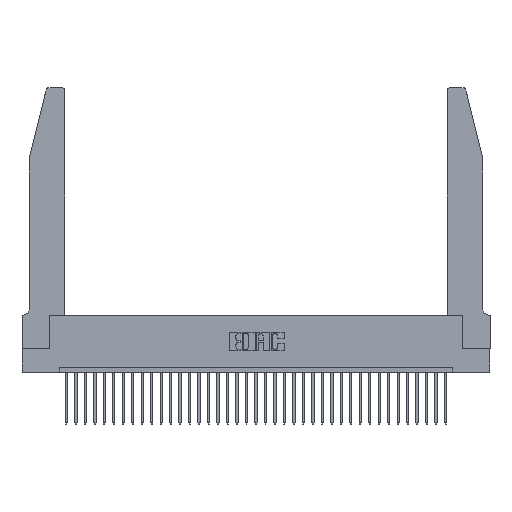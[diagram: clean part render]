
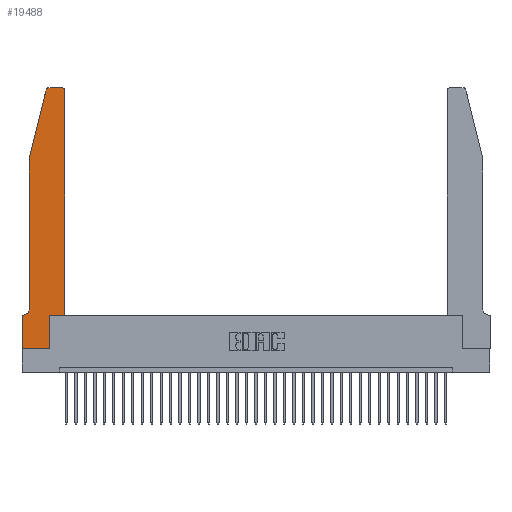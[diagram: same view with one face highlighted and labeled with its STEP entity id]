
A CAD part, top view. The second image highlights one B-rep face of the part: STEP entity #19488.
In plain terms, the highlighted planar face has unit normal (0, 0, 1).
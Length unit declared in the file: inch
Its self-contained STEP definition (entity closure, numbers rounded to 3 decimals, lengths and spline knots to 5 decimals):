
#226 = ORIENTED_EDGE ( 'NONE', *, *, #31575, .T. ) ;
#304 = LINE ( 'NONE', #4262, #28851 ) ;
#483 = LINE ( 'NONE', #24571, #19931 ) ;
#789 = DIRECTION ( 'NONE',  ( -1., 0., 0. ) ) ;
#846 = DIRECTION ( 'NONE',  ( -0.239, -0.971, 0. ) ) ;
#2002 = ORIENTED_EDGE ( 'NONE', *, *, #4133, .T. ) ;
#2169 = LINE ( 'NONE', #10040, #11622 ) ;
#2598 = ORIENTED_EDGE ( 'NONE', *, *, #31284, .T. ) ;
#2631 = CARTESIAN_POINT ( 'NONE',  ( 0., 0., 0.37 ) ) ;
#3411 = VECTOR ( 'NONE', #789, 39.37008 ) ;
#3444 = EDGE_CURVE ( 'NONE', #24111, #4495, #8761, .T. ) ;
#4103 = CARTESIAN_POINT ( 'NONE',  ( 0.2865, 0.35, 0.37 ) ) ;
#4133 = EDGE_CURVE ( 'NONE', #21514, #27555, #483, .T. ) ;
#4262 = CARTESIAN_POINT ( 'NONE',  ( 0.4505, 0.35, 0.37 ) ) ;
#4495 = VERTEX_POINT ( 'NONE', #30017 ) ;
#4595 = CARTESIAN_POINT ( 'NONE',  ( 0., 0., 0.37 ) ) ;
#5075 = VERTEX_POINT ( 'NONE', #26132 ) ;
#5099 = LINE ( 'NONE', #9094, #8101 ) ;
#6666 = DIRECTION ( 'NONE',  ( 0., 0., 1. ) ) ;
#6818 = CARTESIAN_POINT ( 'NONE',  ( 0.0055, 0.35, 0.37 ) ) ;
#7024 = VERTEX_POINT ( 'NONE', #15301 ) ;
#7353 = DIRECTION ( 'NONE',  ( 0., -1., 0. ) ) ;
#7466 = DIRECTION ( 'NONE',  ( 0., 1., 0. ) ) ;
#7699 = DIRECTION ( 'NONE',  ( -1., 0., 0. ) ) ;
#7791 = ORIENTED_EDGE ( 'NONE', *, *, #3444, .T. ) ;
#7918 = LINE ( 'NONE', #12838, #14413 ) ;
#8101 = VECTOR ( 'NONE', #846, 39.37008 ) ;
#8761 = CIRCLE ( 'NONE', #26524, 0.03 ) ;
#9075 = CARTESIAN_POINT ( 'NONE',  ( 0.4205, 2.72, 0.37 ) ) ;
#9094 = CARTESIAN_POINT ( 'NONE',  ( 0.0755, 2., 0.37 ) ) ;
#10027 = CARTESIAN_POINT ( 'NONE',  ( 0.2865, 0.35, 0.37 ) ) ;
#10040 = CARTESIAN_POINT ( 'NONE',  ( 0.0755, 2., 0.37 ) ) ;
#10160 = ORIENTED_EDGE ( 'NONE', *, *, #34799, .T. ) ;
#10247 = DIRECTION ( 'NONE',  ( 0., 0., 1. ) ) ;
#10797 = EDGE_CURVE ( 'NONE', #33736, #19148, #20844, .T. ) ;
#10917 = VERTEX_POINT ( 'NONE', #2631 ) ;
#11254 = CIRCLE ( 'NONE', #30261, 0.03 ) ;
#11622 = VECTOR ( 'NONE', #23765, 39.37008 ) ;
#11906 = DIRECTION ( 'NONE',  ( 1., 0., 0. ) ) ;
#12141 = LINE ( 'NONE', #20479, #3411 ) ;
#12248 = EDGE_LOOP ( 'NONE', ( #10160, #7791, #17104, #32396, #226, #2002, #29447, #19684, #18081, #34953, #2598, #27788 ) ) ;
#12269 = EDGE_CURVE ( 'NONE', #7024, #22123, #2169, .T. ) ;
#12838 = CARTESIAN_POINT ( 'NONE',  ( 0.4505, 0.35, 0.37 ) ) ;
#13035 = CARTESIAN_POINT ( 'NONE',  ( 0., 0., 0.37 ) ) ;
#13229 = EDGE_CURVE ( 'NONE', #4495, #7024, #5099, .T. ) ;
#13727 = VERTEX_POINT ( 'NONE', #34047 ) ;
#14350 = DIRECTION ( 'NONE',  ( 0., 0., -1. ) ) ;
#14394 = AXIS2_PLACEMENT_3D ( 'NONE', #17130, #14350, #30894 ) ;
#14413 = VECTOR ( 'NONE', #35172, 39.37008 ) ;
#14941 = CARTESIAN_POINT ( 'NONE',  ( 0.284, 2.72, 0.37 ) ) ;
#15301 = CARTESIAN_POINT ( 'NONE',  ( 0.0755, 2., 0.37 ) ) ;
#15573 = CARTESIAN_POINT ( 'NONE',  ( 0.4505, 0.35, 0.37 ) ) ;
#16339 = CARTESIAN_POINT ( 'NONE',  ( 0.284, 2.75, 0.37 ) ) ;
#16997 = CARTESIAN_POINT ( 'NONE',  ( 0., 0.35, 0.37 ) ) ;
#17104 = ORIENTED_EDGE ( 'NONE', *, *, #13229, .T. ) ;
#17130 = CARTESIAN_POINT ( 'NONE',  ( 0.0055, 0.42, 0.37 ) ) ;
#17833 = DIRECTION ( 'NONE',  ( 0., 0., 1. ) ) ;
#18081 = ORIENTED_EDGE ( 'NONE', *, *, #10797, .T. ) ;
#18465 = CARTESIAN_POINT ( 'NONE',  ( 0., 0.35, 0.37 ) ) ;
#18677 = CARTESIAN_POINT ( 'NONE',  ( 0.0755, 0.42, 0.37 ) ) ;
#19148 = VERTEX_POINT ( 'NONE', #4103 ) ;
#19488 = ADVANCED_FACE ( 'NONE', ( #25730 ), #29574, .T. ) ;
#19534 = VECTOR ( 'NONE', #7466, 39.37008 ) ;
#19553 = CIRCLE ( 'NONE', #14394, 0.07 ) ;
#19684 = ORIENTED_EDGE ( 'NONE', *, *, #23951, .T. ) ;
#19931 = VECTOR ( 'NONE', #7699, 39.37008 ) ;
#20479 = CARTESIAN_POINT ( 'NONE',  ( 0.2605, 2.75, 0.37 ) ) ;
#20844 = LINE ( 'NONE', #10027, #19534 ) ;
#20922 = DIRECTION ( 'NONE',  ( 1., 0., 0. ) ) ;
#21252 = LINE ( 'NONE', #4595, #21692 ) ;
#21514 = VERTEX_POINT ( 'NONE', #6818 ) ;
#21692 = VECTOR ( 'NONE', #7353, 39.37008 ) ;
#21945 = EDGE_CURVE ( 'NONE', #19148, #30232, #304, .T. ) ;
#22123 = VERTEX_POINT ( 'NONE', #18677 ) ;
#23765 = DIRECTION ( 'NONE',  ( 0., -1., 0. ) ) ;
#23951 = EDGE_CURVE ( 'NONE', #10917, #33736, #28734, .T. ) ;
#24111 = VERTEX_POINT ( 'NONE', #16339 ) ;
#24500 = CARTESIAN_POINT ( 'NONE',  ( 0.2865, 0., 0.37 ) ) ;
#24571 = CARTESIAN_POINT ( 'NONE',  ( 0.0755, 0.35, 0.37 ) ) ;
#25613 = DIRECTION ( 'NONE',  ( 1., 0., 0. ) ) ;
#25730 = FACE_OUTER_BOUND ( 'NONE', #12248, .T. ) ;
#26132 = CARTESIAN_POINT ( 'NONE',  ( 0.4205, 2.75, 0.37 ) ) ;
#26375 = EDGE_CURVE ( 'NONE', #27555, #10917, #21252, .T. ) ;
#26524 = AXIS2_PLACEMENT_3D ( 'NONE', #14941, #17833, #11906 ) ;
#26672 = DIRECTION ( 'NONE',  ( 1., 0., 0. ) ) ;
#27224 = EDGE_CURVE ( 'NONE', #13727, #5075, #11254, .T. ) ;
#27555 = VERTEX_POINT ( 'NONE', #16997 ) ;
#27788 = ORIENTED_EDGE ( 'NONE', *, *, #27224, .T. ) ;
#28734 = LINE ( 'NONE', #13035, #35245 ) ;
#28851 = VECTOR ( 'NONE', #20922, 39.37008 ) ;
#29447 = ORIENTED_EDGE ( 'NONE', *, *, #26375, .T. ) ;
#29574 = PLANE ( 'NONE',  #35199 ) ;
#30017 = CARTESIAN_POINT ( 'NONE',  ( 0.25487, 2.72718, 0.37 ) ) ;
#30232 = VERTEX_POINT ( 'NONE', #15573 ) ;
#30261 = AXIS2_PLACEMENT_3D ( 'NONE', #9075, #6666, #25613 ) ;
#30894 = DIRECTION ( 'NONE',  ( -1., 0., 0. ) ) ;
#31284 = EDGE_CURVE ( 'NONE', #30232, #13727, #7918, .T. ) ;
#31575 = EDGE_CURVE ( 'NONE', #22123, #21514, #19553, .T. ) ;
#32396 = ORIENTED_EDGE ( 'NONE', *, *, #12269, .T. ) ;
#33736 = VERTEX_POINT ( 'NONE', #24500 ) ;
#34047 = CARTESIAN_POINT ( 'NONE',  ( 0.4505, 2.72, 0.37 ) ) ;
#34799 = EDGE_CURVE ( 'NONE', #5075, #24111, #12141, .T. ) ;
#34893 = DIRECTION ( 'NONE',  ( 1., 0., 0. ) ) ;
#34953 = ORIENTED_EDGE ( 'NONE', *, *, #21945, .T. ) ;
#35172 = DIRECTION ( 'NONE',  ( 0., 1., 0. ) ) ;
#35199 = AXIS2_PLACEMENT_3D ( 'NONE', #18465, #10247, #34893 ) ;
#35245 = VECTOR ( 'NONE', #26672, 39.37008 ) ;
